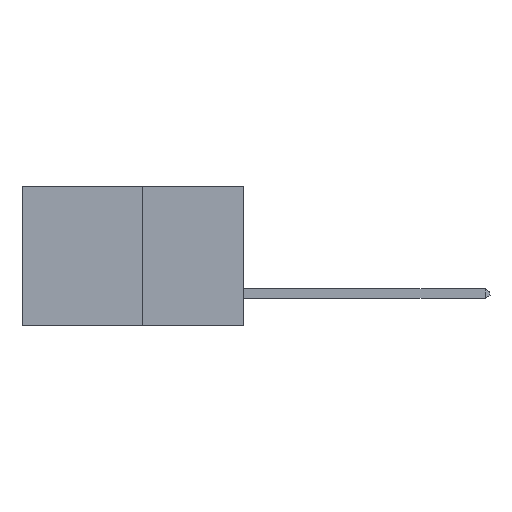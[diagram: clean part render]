
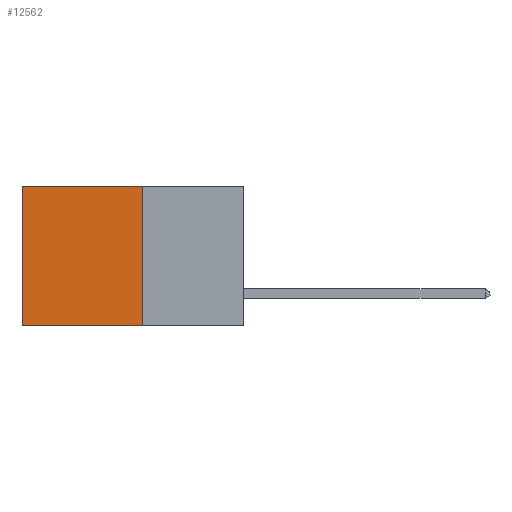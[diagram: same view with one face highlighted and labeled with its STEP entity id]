
A CAD part, left-side view. The second image highlights one B-rep face of the part: STEP entity #12562.
In plain terms, the highlighted planar face has unit normal (-1, 0, 0).
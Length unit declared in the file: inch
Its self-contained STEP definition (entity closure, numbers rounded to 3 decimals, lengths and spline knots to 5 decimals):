
#86 = CARTESIAN_POINT ( 'NONE',  ( 0.277, 0.59, 0. ) ) ;
#451 = FACE_OUTER_BOUND ( 'NONE', #10176, .T. ) ;
#1035 = AXIS2_PLACEMENT_3D ( 'NONE', #2176, #10325, #4261 ) ;
#1136 = PLANE ( 'NONE',  #1035 ) ;
#1338 = VECTOR ( 'NONE', #12900, 39.37008 ) ;
#2153 = CARTESIAN_POINT ( 'NONE',  ( 0.277, 0.59, -0.37 ) ) ;
#2176 = CARTESIAN_POINT ( 'NONE',  ( 0.277, 0.27, -0.37 ) ) ;
#2453 = VECTOR ( 'NONE', #6535, 39.37008 ) ;
#3132 = VECTOR ( 'NONE', #4034, 39.37008 ) ;
#3904 = CARTESIAN_POINT ( 'NONE',  ( 0.277, 0.27, -0.37 ) ) ;
#4034 = DIRECTION ( 'NONE',  ( 0., 1., 0. ) ) ;
#4261 = DIRECTION ( 'NONE',  ( 0., 0., -1. ) ) ;
#4826 = ORIENTED_EDGE ( 'NONE', *, *, #10838, .F. ) ;
#5412 = EDGE_CURVE ( 'NONE', #10830, #9599, #7099, .T. ) ;
#5701 = CARTESIAN_POINT ( 'NONE',  ( 0.277, 0.27, -0.37 ) ) ;
#6330 = DIRECTION ( 'NONE',  ( 0., 1., 0. ) ) ;
#6535 = DIRECTION ( 'NONE',  ( 0., 0., -1. ) ) ;
#6620 = VECTOR ( 'NONE', #6330, 39.37008 ) ;
#6931 = LINE ( 'NONE', #11345, #6620 ) ;
#7099 = LINE ( 'NONE', #3904, #1338 ) ;
#7788 = ORIENTED_EDGE ( 'NONE', *, *, #10332, .T. ) ;
#9136 = CARTESIAN_POINT ( 'NONE',  ( 0.277, 0.27, 0. ) ) ;
#9324 = VERTEX_POINT ( 'NONE', #2153 ) ;
#9382 = CARTESIAN_POINT ( 'NONE',  ( 0.277, 0.27, 0. ) ) ;
#9599 = VERTEX_POINT ( 'NONE', #5701 ) ;
#9850 = EDGE_CURVE ( 'NONE', #10830, #10802, #10612, .T. ) ;
#10176 = EDGE_LOOP ( 'NONE', ( #7788, #4826, #11286, #12767 ) ) ;
#10266 = LINE ( 'NONE', #12526, #2453 ) ;
#10325 = DIRECTION ( 'NONE',  ( 1., 0., 0. ) ) ;
#10332 = EDGE_CURVE ( 'NONE', #10802, #9324, #10266, .T. ) ;
#10612 = LINE ( 'NONE', #9136, #3132 ) ;
#10802 = VERTEX_POINT ( 'NONE', #86 ) ;
#10830 = VERTEX_POINT ( 'NONE', #9382 ) ;
#10838 = EDGE_CURVE ( 'NONE', #9599, #9324, #6931, .T. ) ;
#11286 = ORIENTED_EDGE ( 'NONE', *, *, #5412, .F. ) ;
#11345 = CARTESIAN_POINT ( 'NONE',  ( 0.277, 0.27, -0.37 ) ) ;
#12526 = CARTESIAN_POINT ( 'NONE',  ( 0.277, 0.59, -0.37 ) ) ;
#12562 = ADVANCED_FACE ( 'NONE', ( #451 ), #1136, .F. ) ;
#12767 = ORIENTED_EDGE ( 'NONE', *, *, #9850, .T. ) ;
#12900 = DIRECTION ( 'NONE',  ( 0., 0., -1. ) ) ;
